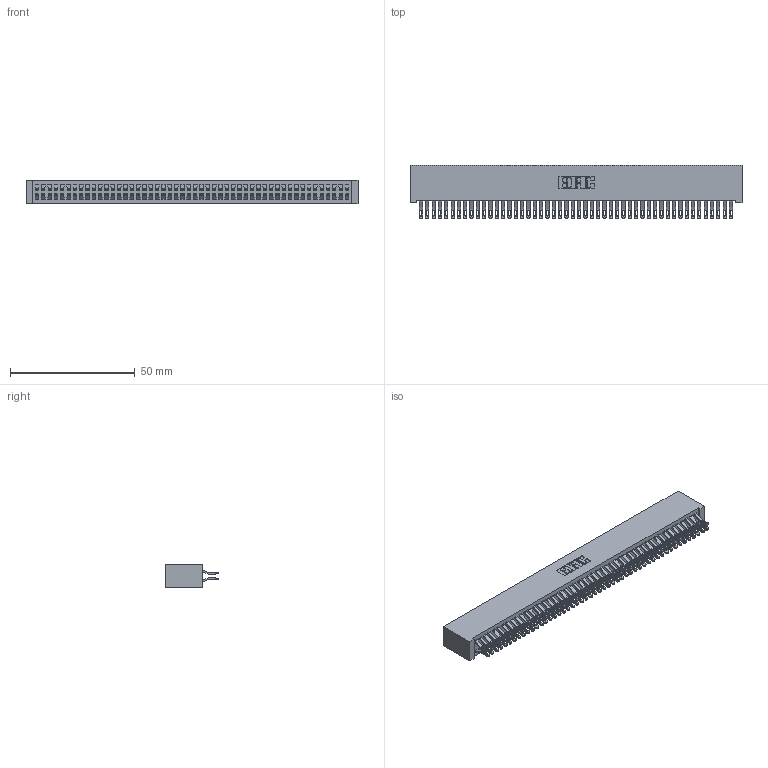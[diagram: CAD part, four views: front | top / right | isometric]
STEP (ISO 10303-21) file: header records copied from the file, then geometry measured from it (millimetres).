
FILE_DESCRIPTION (( 'STEP AP203' ), '1' );
FILE_NAME ('342-100-555-201.STEP', '2018-08-14T04:45:48', ( '' ), ( '' ), 'SwSTEP 2.0', 'SolidWorks 2016', '' );
FILE_SCHEMA (( 'CONFIG_CONTROL_DESIGN' ));
Length unit declared in the file: inch
Products named in the file (3): 342 Part_Lugless; 345-292-001_555 Tail; 342-100-555-201
Assembly tree (101 placements, depth 2):
  342-100-555-201
    342 Part_Lugless
    345-292-001_555 Tail  x100
Bounding box: 133.25 x 21.47 x 9.4 mm (x, y, z)
Volume: 12727.6 mm3; surface area: 22328.3 mm2
Topology: 101 solids, 101 shells, 5902 faces, 18575 edges, 12382 vertices
Faces by surface type: plane 3462, cylinder 2440
Entity records: 31049 total; most frequent: CARTESIAN_POINT 5168, ORIENTED_EDGE 5074, DIRECTION 4365, EDGE_CURVE 2537, VECTOR 2397, LINE 2397, VERTEX_POINT 1690, AXIS2_PLACEMENT_3D 984
